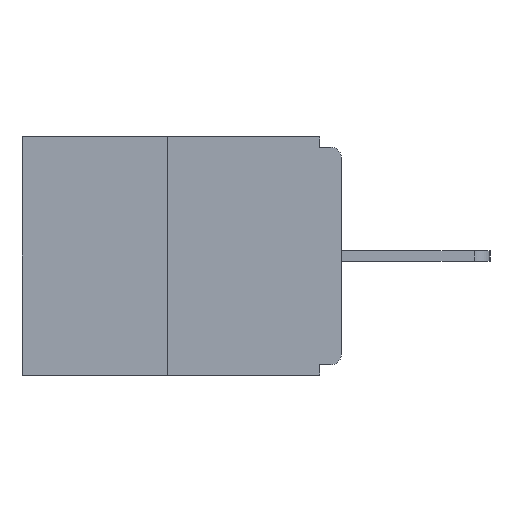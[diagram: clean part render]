
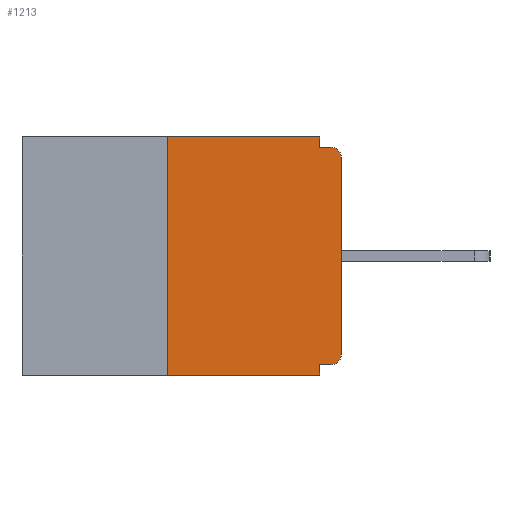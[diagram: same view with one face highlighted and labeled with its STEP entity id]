
A CAD part, left-side view. The second image highlights one B-rep face of the part: STEP entity #1213.
In plain terms, the highlighted planar face has unit normal (-1, 0, 0).
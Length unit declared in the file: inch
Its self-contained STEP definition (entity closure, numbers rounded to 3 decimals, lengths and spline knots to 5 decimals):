
#185 = VERTEX_POINT ( 'NONE', #11781 ) ;
#239 = DIRECTION ( 'NONE',  ( 0., -1., 0. ) ) ;
#470 = EDGE_CURVE ( 'NONE', #11326, #807, #4321, .T. ) ;
#559 = EDGE_CURVE ( 'NONE', #10939, #807, #6033, .T. ) ;
#666 = DIRECTION ( 'NONE',  ( 0., 0., -1. ) ) ;
#713 = AXIS2_PLACEMENT_3D ( 'NONE', #12880, #6299, #13959 ) ;
#727 = CARTESIAN_POINT ( 'NONE',  ( 0., 0.015, -0.328 ) ) ;
#785 = CARTESIAN_POINT ( 'NONE',  ( 0., 0.031, 0. ) ) ;
#807 = VERTEX_POINT ( 'NONE', #1353 ) ;
#873 = EDGE_CURVE ( 'NONE', #12649, #2098, #11066, .T. ) ;
#876 = VECTOR ( 'NONE', #10347, 39.37008 ) ;
#985 = ORIENTED_EDGE ( 'NONE', *, *, #14620, .T. ) ;
#1165 = VECTOR ( 'NONE', #12316, 39.37008 ) ;
#1213 = ADVANCED_FACE ( 'NONE', ( #4124 ), #5397, .F. ) ;
#1353 = CARTESIAN_POINT ( 'NONE',  ( 0., 0.031, -0.343 ) ) ;
#1549 = VERTEX_POINT ( 'NONE', #9384 ) ;
#1599 = CARTESIAN_POINT ( 'NONE',  ( 0., 0., 0. ) ) ;
#1744 = ORIENTED_EDGE ( 'NONE', *, *, #873, .F. ) ;
#2098 = VERTEX_POINT ( 'NONE', #13976 ) ;
#3141 = VERTEX_POINT ( 'NONE', #10742 ) ;
#3340 = CARTESIAN_POINT ( 'NONE',  ( 0., 0., -0.015 ) ) ;
#3600 = VECTOR ( 'NONE', #8806, 39.37008 ) ;
#3765 = EDGE_CURVE ( 'NONE', #11990, #10939, #10348, .T. ) ;
#4102 = LINE ( 'NONE', #8604, #12722 ) ;
#4124 = FACE_OUTER_BOUND ( 'NONE', #4317, .T. ) ;
#4244 = AXIS2_PLACEMENT_3D ( 'NONE', #11752, #5021, #12839 ) ;
#4317 = EDGE_LOOP ( 'NONE', ( #5388, #11332, #5755, #6522, #12337, #9851, #985, #13019, #7590, #1744 ) ) ;
#4321 = LINE ( 'NONE', #8573, #876 ) ;
#5021 = DIRECTION ( 'NONE',  ( -1., 0., 0. ) ) ;
#5149 = CIRCLE ( 'NONE', #713, 0.015 ) ;
#5385 = DIRECTION ( 'NONE',  ( 1., 0., 0. ) ) ;
#5388 = ORIENTED_EDGE ( 'NONE', *, *, #8811, .F. ) ;
#5397 = PLANE ( 'NONE',  #10599 ) ;
#5399 = CARTESIAN_POINT ( 'NONE',  ( 0., 0.46, 0. ) ) ;
#5755 = ORIENTED_EDGE ( 'NONE', *, *, #470, .T. ) ;
#5877 = DIRECTION ( 'NONE',  ( 0., 0., -1. ) ) ;
#6033 = LINE ( 'NONE', #13657, #3600 ) ;
#6114 = LINE ( 'NONE', #3340, #11973 ) ;
#6299 = DIRECTION ( 'NONE',  ( -1., 0., 0. ) ) ;
#6522 = ORIENTED_EDGE ( 'NONE', *, *, #559, .F. ) ;
#6598 = CARTESIAN_POINT ( 'NONE',  ( 0., 0., -0.03 ) ) ;
#6711 = CARTESIAN_POINT ( 'NONE',  ( 0., 0.031, -0.328 ) ) ;
#7583 = CARTESIAN_POINT ( 'NONE',  ( 0., 0.25, -0.343 ) ) ;
#7590 = ORIENTED_EDGE ( 'NONE', *, *, #13056, .F. ) ;
#7728 = EDGE_CURVE ( 'NONE', #11990, #1549, #8519, .T. ) ;
#8044 = LINE ( 'NONE', #1599, #13801 ) ;
#8163 = VECTOR ( 'NONE', #666, 39.37008 ) ;
#8519 = CIRCLE ( 'NONE', #4244, 0.015 ) ;
#8573 = CARTESIAN_POINT ( 'NONE',  ( 0., 0.46, -0.343 ) ) ;
#8604 = CARTESIAN_POINT ( 'NONE',  ( 0., 0.25, 0. ) ) ;
#8806 = DIRECTION ( 'NONE',  ( 0., 0., -1. ) ) ;
#8811 = EDGE_CURVE ( 'NONE', #185, #12649, #9368, .T. ) ;
#8976 = EDGE_CURVE ( 'NONE', #11326, #185, #4102, .T. ) ;
#9074 = VERTEX_POINT ( 'NONE', #6598 ) ;
#9368 = LINE ( 'NONE', #13786, #11869 ) ;
#9384 = CARTESIAN_POINT ( 'NONE',  ( 0., 0., -0.313 ) ) ;
#9765 = DIRECTION ( 'NONE',  ( 0., 0., 1. ) ) ;
#9851 = ORIENTED_EDGE ( 'NONE', *, *, #7728, .T. ) ;
#10347 = DIRECTION ( 'NONE',  ( 0., -1., 0. ) ) ;
#10348 = LINE ( 'NONE', #13081, #1165 ) ;
#10599 = AXIS2_PLACEMENT_3D ( 'NONE', #5399, #5385, #5877 ) ;
#10742 = CARTESIAN_POINT ( 'NONE',  ( 0., 0.015, -0.015 ) ) ;
#10939 = VERTEX_POINT ( 'NONE', #6711 ) ;
#11066 = LINE ( 'NONE', #785, #8163 ) ;
#11283 = DIRECTION ( 'NONE',  ( 0., -1., 0. ) ) ;
#11326 = VERTEX_POINT ( 'NONE', #7583 ) ;
#11332 = ORIENTED_EDGE ( 'NONE', *, *, #8976, .F. ) ;
#11752 = CARTESIAN_POINT ( 'NONE',  ( 0., 0.015, -0.313 ) ) ;
#11781 = CARTESIAN_POINT ( 'NONE',  ( 0., 0.25, 0. ) ) ;
#11802 = DIRECTION ( 'NONE',  ( 0., 0., 1. ) ) ;
#11869 = VECTOR ( 'NONE', #239, 39.37008 ) ;
#11973 = VECTOR ( 'NONE', #11283, 39.37008 ) ;
#11990 = VERTEX_POINT ( 'NONE', #727 ) ;
#12316 = DIRECTION ( 'NONE',  ( 0., 1., 0. ) ) ;
#12322 = CARTESIAN_POINT ( 'NONE',  ( 0., 0.031, 0. ) ) ;
#12337 = ORIENTED_EDGE ( 'NONE', *, *, #3765, .F. ) ;
#12649 = VERTEX_POINT ( 'NONE', #12322 ) ;
#12722 = VECTOR ( 'NONE', #9765, 39.37008 ) ;
#12839 = DIRECTION ( 'NONE',  ( 0., 0., -1. ) ) ;
#12880 = CARTESIAN_POINT ( 'NONE',  ( 0., 0.015, -0.03 ) ) ;
#13019 = ORIENTED_EDGE ( 'NONE', *, *, #13387, .T. ) ;
#13056 = EDGE_CURVE ( 'NONE', #2098, #3141, #6114, .T. ) ;
#13081 = CARTESIAN_POINT ( 'NONE',  ( 0., 0., -0.328 ) ) ;
#13387 = EDGE_CURVE ( 'NONE', #9074, #3141, #5149, .T. ) ;
#13657 = CARTESIAN_POINT ( 'NONE',  ( 0., 0.031, -0.343 ) ) ;
#13786 = CARTESIAN_POINT ( 'NONE',  ( 0., 0.46, 0. ) ) ;
#13801 = VECTOR ( 'NONE', #11802, 39.37008 ) ;
#13959 = DIRECTION ( 'NONE',  ( 0., 0., -1. ) ) ;
#13976 = CARTESIAN_POINT ( 'NONE',  ( 0., 0.031, -0.015 ) ) ;
#14620 = EDGE_CURVE ( 'NONE', #1549, #9074, #8044, .T. ) ;
